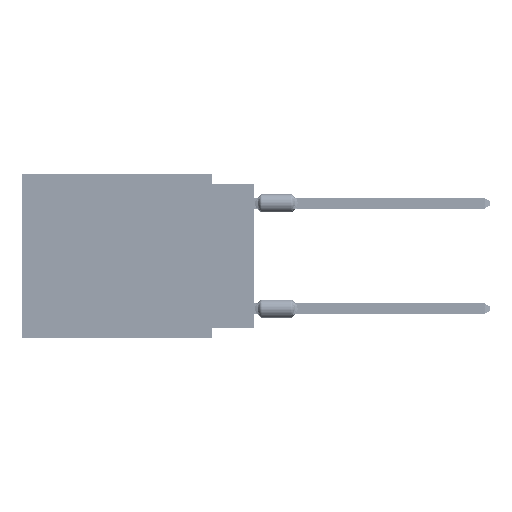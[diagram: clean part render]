
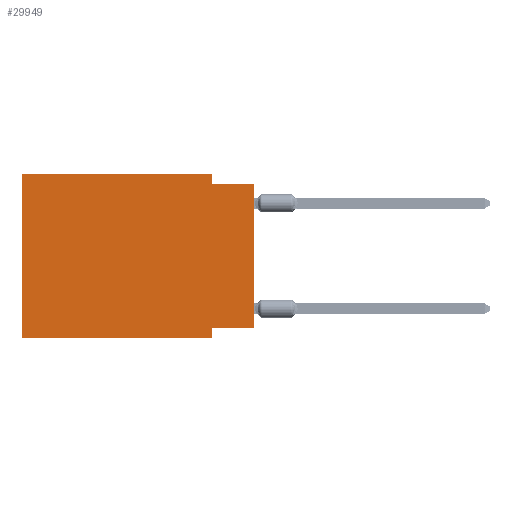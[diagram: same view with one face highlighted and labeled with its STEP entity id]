
A CAD part, left-side view. The second image highlights one B-rep face of the part: STEP entity #29949.
In plain terms, the highlighted planar face has unit normal (-1, 0, 0).
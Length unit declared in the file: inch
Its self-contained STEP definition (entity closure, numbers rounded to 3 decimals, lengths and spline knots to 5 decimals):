
#158 = CARTESIAN_POINT ( 'NONE',  ( 0., 0.1, -0.39 ) ) ;
#1279 = VECTOR ( 'NONE', #16302, 39.37008 ) ;
#2189 = VERTEX_POINT ( 'NONE', #76460 ) ;
#2614 = ORIENTED_EDGE ( 'NONE', *, *, #73233, .F. ) ;
#3159 = CARTESIAN_POINT ( 'NONE',  ( 0., 0.1, 0. ) ) ;
#3329 = CARTESIAN_POINT ( 'NONE',  ( 0., 0., -0.365 ) ) ;
#3399 = DIRECTION ( 'NONE',  ( 0., 0., -1. ) ) ;
#5285 = DIRECTION ( 'NONE',  ( 0., 0., -1. ) ) ;
#7044 = VERTEX_POINT ( 'NONE', #71974 ) ;
#7632 = VECTOR ( 'NONE', #29643, 39.37008 ) ;
#7940 = VECTOR ( 'NONE', #55859, 39.37008 ) ;
#9590 = ORIENTED_EDGE ( 'NONE', *, *, #67449, .F. ) ;
#12055 = CARTESIAN_POINT ( 'NONE',  ( 0., 0.55, 0. ) ) ;
#13755 = CARTESIAN_POINT ( 'NONE',  ( 0., 0.1, -0.025 ) ) ;
#15125 = VECTOR ( 'NONE', #45376, 39.37008 ) ;
#16232 = CARTESIAN_POINT ( 'NONE',  ( 0., 0.55, 0. ) ) ;
#16302 = DIRECTION ( 'NONE',  ( 0., -1., 0. ) ) ;
#16634 = CARTESIAN_POINT ( 'NONE',  ( 0., 0.55, -0.39 ) ) ;
#17780 = CARTESIAN_POINT ( 'NONE',  ( 0., 0.1, 0. ) ) ;
#19995 = EDGE_CURVE ( 'NONE', #57316, #2189, #29583, .T. ) ;
#20965 = VECTOR ( 'NONE', #76106, 39.37008 ) ;
#21814 = DIRECTION ( 'NONE',  ( 1., 0., 0. ) ) ;
#21895 = LINE ( 'NONE', #54344, #1279 ) ;
#23482 = PLANE ( 'NONE',  #46500 ) ;
#25946 = EDGE_LOOP ( 'NONE', ( #30604, #76806, #82122, #2614, #51442, #80604, #49294, #9590 ) ) ;
#29300 = EDGE_CURVE ( 'NONE', #7044, #49532, #37745, .T. ) ;
#29583 = LINE ( 'NONE', #30424, #59575 ) ;
#29643 = DIRECTION ( 'NONE',  ( 0., 0., -1. ) ) ;
#29949 = ADVANCED_FACE ( 'NONE', ( #67932 ), #23482, .F. ) ;
#30424 = CARTESIAN_POINT ( 'NONE',  ( 0., 0., 0. ) ) ;
#30604 = ORIENTED_EDGE ( 'NONE', *, *, #19995, .T. ) ;
#36534 = CARTESIAN_POINT ( 'NONE',  ( 0., 0., -0.365 ) ) ;
#37647 = VECTOR ( 'NONE', #44872, 39.37008 ) ;
#37745 = LINE ( 'NONE', #158, #69539 ) ;
#38462 = LINE ( 'NONE', #52544, #37647 ) ;
#38928 = VERTEX_POINT ( 'NONE', #17780 ) ;
#39774 = EDGE_CURVE ( 'NONE', #44832, #65167, #64119, .T. ) ;
#43046 = LINE ( 'NONE', #3329, #7940 ) ;
#43084 = EDGE_CURVE ( 'NONE', #68536, #2189, #38462, .T. ) ;
#44832 = VERTEX_POINT ( 'NONE', #16634 ) ;
#44872 = DIRECTION ( 'NONE',  ( 0., -1., 0. ) ) ;
#45376 = DIRECTION ( 'NONE',  ( 0., -1., 0. ) ) ;
#46500 = AXIS2_PLACEMENT_3D ( 'NONE', #16232, #21814, #3399 ) ;
#49294 = ORIENTED_EDGE ( 'NONE', *, *, #29300, .F. ) ;
#49532 = VERTEX_POINT ( 'NONE', #76265 ) ;
#51442 = ORIENTED_EDGE ( 'NONE', *, *, #39774, .F. ) ;
#52544 = CARTESIAN_POINT ( 'NONE',  ( 0., 0., -0.025 ) ) ;
#54344 = CARTESIAN_POINT ( 'NONE',  ( 0., 0.55, -0.39 ) ) ;
#55859 = DIRECTION ( 'NONE',  ( 0., 1., 0. ) ) ;
#57316 = VERTEX_POINT ( 'NONE', #36534 ) ;
#59575 = VECTOR ( 'NONE', #63721, 39.37008 ) ;
#62296 = CARTESIAN_POINT ( 'NONE',  ( 0., 0.55, 0. ) ) ;
#62504 = LINE ( 'NONE', #3159, #7632 ) ;
#63721 = DIRECTION ( 'NONE',  ( 0., 0., 1. ) ) ;
#64119 = LINE ( 'NONE', #82945, #20965 ) ;
#64583 = LINE ( 'NONE', #12055, #15125 ) ;
#65167 = VERTEX_POINT ( 'NONE', #62296 ) ;
#65476 = EDGE_CURVE ( 'NONE', #38928, #68536, #62504, .T. ) ;
#67449 = EDGE_CURVE ( 'NONE', #57316, #7044, #43046, .T. ) ;
#67932 = FACE_OUTER_BOUND ( 'NONE', #25946, .T. ) ;
#68536 = VERTEX_POINT ( 'NONE', #13755 ) ;
#69539 = VECTOR ( 'NONE', #5285, 39.37008 ) ;
#71974 = CARTESIAN_POINT ( 'NONE',  ( 0., 0.1, -0.365 ) ) ;
#73233 = EDGE_CURVE ( 'NONE', #65167, #38928, #64583, .T. ) ;
#76106 = DIRECTION ( 'NONE',  ( 0., 0., 1. ) ) ;
#76265 = CARTESIAN_POINT ( 'NONE',  ( 0., 0.1, -0.39 ) ) ;
#76460 = CARTESIAN_POINT ( 'NONE',  ( 0., 0., -0.025 ) ) ;
#76806 = ORIENTED_EDGE ( 'NONE', *, *, #43084, .F. ) ;
#80604 = ORIENTED_EDGE ( 'NONE', *, *, #82578, .T. ) ;
#82122 = ORIENTED_EDGE ( 'NONE', *, *, #65476, .F. ) ;
#82578 = EDGE_CURVE ( 'NONE', #44832, #49532, #21895, .T. ) ;
#82945 = CARTESIAN_POINT ( 'NONE',  ( 0., 0.55, 0. ) ) ;
